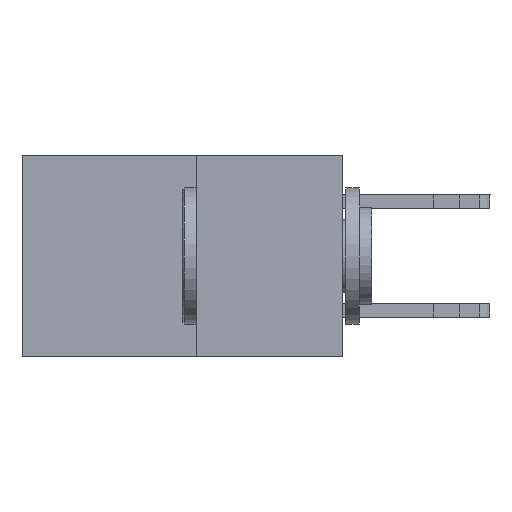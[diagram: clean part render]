
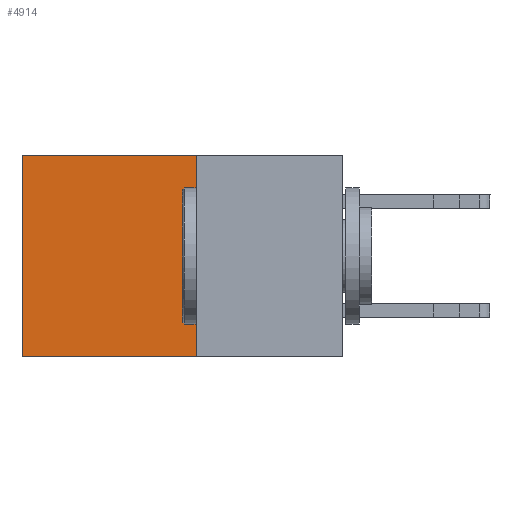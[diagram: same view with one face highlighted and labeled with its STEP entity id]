
A CAD part, left-side view. The second image highlights one B-rep face of the part: STEP entity #4914.
In plain terms, the highlighted planar face has unit normal (-1, 0, 0).
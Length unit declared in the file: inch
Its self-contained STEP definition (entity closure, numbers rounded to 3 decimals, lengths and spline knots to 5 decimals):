
#270 = VECTOR ( 'NONE', #16710, 39.37008 ) ;
#791 = ORIENTED_EDGE ( 'NONE', *, *, #9509, .T. ) ;
#1263 = AXIS2_PLACEMENT_3D ( 'NONE', #8555, #3408, #1929 ) ;
#1929 = DIRECTION ( 'NONE',  ( 0., 0., -1. ) ) ;
#2012 = VECTOR ( 'NONE', #17554, 39.37008 ) ;
#2136 = PLANE ( 'NONE',  #1263 ) ;
#2888 = DIRECTION ( 'NONE',  ( 0., 1., 0. ) ) ;
#3318 = CARTESIAN_POINT ( 'NONE',  ( 0.277, 0.59, 0. ) ) ;
#3408 = DIRECTION ( 'NONE',  ( 1., 0., 0. ) ) ;
#4109 = ORIENTED_EDGE ( 'NONE', *, *, #15075, .T. ) ;
#4914 = ADVANCED_FACE ( 'NONE', ( #16358 ), #2136, .F. ) ;
#5125 = LINE ( 'NONE', #13017, #2012 ) ;
#5325 = CARTESIAN_POINT ( 'NONE',  ( 0.277, 0.27, 0. ) ) ;
#6160 = EDGE_CURVE ( 'NONE', #14833, #8465, #12483, .T. ) ;
#7220 = LINE ( 'NONE', #7333, #270 ) ;
#7333 = CARTESIAN_POINT ( 'NONE',  ( 0.277, 0.27, -0.37 ) ) ;
#7639 = ORIENTED_EDGE ( 'NONE', *, *, #6160, .F. ) ;
#7720 = EDGE_LOOP ( 'NONE', ( #791, #15743, #7639, #4109 ) ) ;
#7933 = CARTESIAN_POINT ( 'NONE',  ( 0.277, 0.27, -0.37 ) ) ;
#8465 = VERTEX_POINT ( 'NONE', #10247 ) ;
#8555 = CARTESIAN_POINT ( 'NONE',  ( 0.277, 0.27, -0.37 ) ) ;
#9509 = EDGE_CURVE ( 'NONE', #9803, #16874, #5125, .T. ) ;
#9803 = VERTEX_POINT ( 'NONE', #3318 ) ;
#10247 = CARTESIAN_POINT ( 'NONE',  ( 0.277, 0.27, -0.37 ) ) ;
#10919 = VECTOR ( 'NONE', #2888, 39.37008 ) ;
#11005 = DIRECTION ( 'NONE',  ( 0., 0., -1. ) ) ;
#12483 = LINE ( 'NONE', #7933, #17083 ) ;
#13017 = CARTESIAN_POINT ( 'NONE',  ( 0.277, 0.59, -0.37 ) ) ;
#13344 = LINE ( 'NONE', #13844, #10919 ) ;
#13844 = CARTESIAN_POINT ( 'NONE',  ( 0.277, 0.27, 0. ) ) ;
#14833 = VERTEX_POINT ( 'NONE', #5325 ) ;
#15075 = EDGE_CURVE ( 'NONE', #14833, #9803, #13344, .T. ) ;
#15336 = CARTESIAN_POINT ( 'NONE',  ( 0.277, 0.59, -0.37 ) ) ;
#15743 = ORIENTED_EDGE ( 'NONE', *, *, #16769, .F. ) ;
#16358 = FACE_OUTER_BOUND ( 'NONE', #7720, .T. ) ;
#16710 = DIRECTION ( 'NONE',  ( 0., 1., 0. ) ) ;
#16769 = EDGE_CURVE ( 'NONE', #8465, #16874, #7220, .T. ) ;
#16874 = VERTEX_POINT ( 'NONE', #15336 ) ;
#17083 = VECTOR ( 'NONE', #11005, 39.37008 ) ;
#17554 = DIRECTION ( 'NONE',  ( 0., 0., -1. ) ) ;
